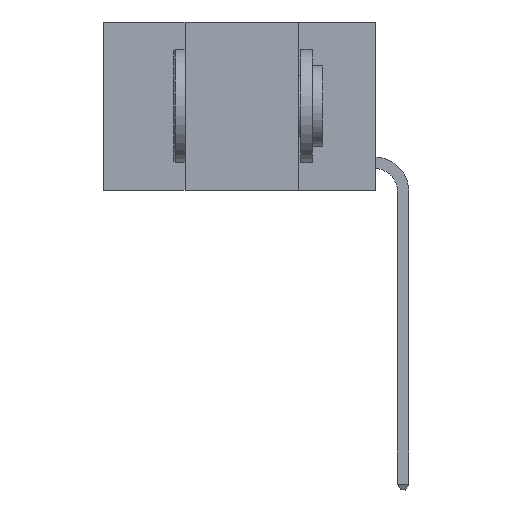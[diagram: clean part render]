
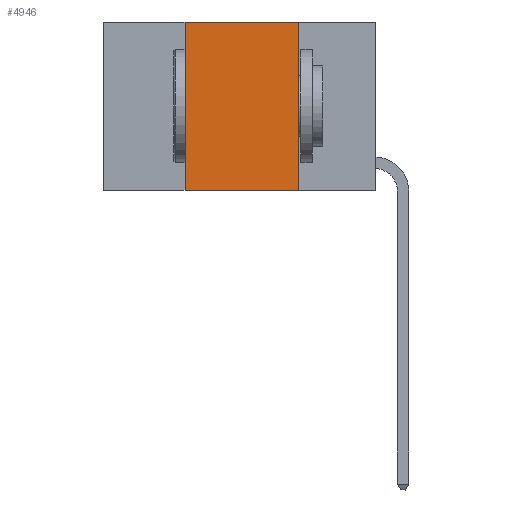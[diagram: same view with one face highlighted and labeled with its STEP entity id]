
A CAD part, left-side view. The second image highlights one B-rep face of the part: STEP entity #4946.
In plain terms, the highlighted planar face has unit normal (-1, 0, 0).
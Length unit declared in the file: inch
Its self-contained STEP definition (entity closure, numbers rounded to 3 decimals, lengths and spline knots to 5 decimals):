
#1655 = CARTESIAN_POINT ( 'NONE',  ( 0., 0.17, 0. ) ) ;
#1860 = AXIS2_PLACEMENT_3D ( 'NONE', #11773, #8439, #4519 ) ;
#2201 = VERTEX_POINT ( 'NONE', #23455 ) ;
#2501 = ORIENTED_EDGE ( 'NONE', *, *, #7021, .F. ) ;
#3033 = DIRECTION ( 'NONE',  ( 0., 0., -1. ) ) ;
#4519 = DIRECTION ( 'NONE',  ( 0., 0., -1. ) ) ;
#4595 = CARTESIAN_POINT ( 'NONE',  ( 0., 0.42, -0.37 ) ) ;
#4626 = FACE_OUTER_BOUND ( 'NONE', #23109, .T. ) ;
#4946 = ADVANCED_FACE ( 'NONE', ( #4626 ), #21467, .F. ) ;
#5181 = VERTEX_POINT ( 'NONE', #4595 ) ;
#6575 = DIRECTION ( 'NONE',  ( 0., -1., 0. ) ) ;
#7021 = EDGE_CURVE ( 'NONE', #2201, #10026, #11549, .T. ) ;
#8439 = DIRECTION ( 'NONE',  ( 1., 0., 0. ) ) ;
#10026 = VERTEX_POINT ( 'NONE', #1655 ) ;
#10428 = LINE ( 'NONE', #23685, #12687 ) ;
#11549 = LINE ( 'NONE', #13533, #18004 ) ;
#11654 = DIRECTION ( 'NONE',  ( 0., -1., 0. ) ) ;
#11773 = CARTESIAN_POINT ( 'NONE',  ( 0., 0.6, 0. ) ) ;
#12687 = VECTOR ( 'NONE', #3033, 39.37008 ) ;
#13533 = CARTESIAN_POINT ( 'NONE',  ( 0., 0.6, 0. ) ) ;
#13561 = VERTEX_POINT ( 'NONE', #16220 ) ;
#15503 = LINE ( 'NONE', #23175, #23399 ) ;
#15741 = VECTOR ( 'NONE', #23298, 39.37008 ) ;
#16220 = CARTESIAN_POINT ( 'NONE',  ( 0., 0.17, -0.37 ) ) ;
#16746 = LINE ( 'NONE', #22428, #15741 ) ;
#16990 = ORIENTED_EDGE ( 'NONE', *, *, #20769, .F. ) ;
#18004 = VECTOR ( 'NONE', #11654, 39.37008 ) ;
#20769 = EDGE_CURVE ( 'NONE', #10026, #13561, #10428, .T. ) ;
#21467 = PLANE ( 'NONE',  #1860 ) ;
#22025 = EDGE_CURVE ( 'NONE', #5181, #13561, #15503, .T. ) ;
#22428 = CARTESIAN_POINT ( 'NONE',  ( 0., 0.42, 0. ) ) ;
#23109 = EDGE_LOOP ( 'NONE', ( #16990, #2501, #23187, #23357 ) ) ;
#23175 = CARTESIAN_POINT ( 'NONE',  ( 0., 0.6, -0.37 ) ) ;
#23187 = ORIENTED_EDGE ( 'NONE', *, *, #23378, .F. ) ;
#23298 = DIRECTION ( 'NONE',  ( 0., 0., 1. ) ) ;
#23357 = ORIENTED_EDGE ( 'NONE', *, *, #22025, .T. ) ;
#23378 = EDGE_CURVE ( 'NONE', #5181, #2201, #16746, .T. ) ;
#23399 = VECTOR ( 'NONE', #6575, 39.37008 ) ;
#23455 = CARTESIAN_POINT ( 'NONE',  ( 0., 0.42, 0. ) ) ;
#23685 = CARTESIAN_POINT ( 'NONE',  ( 0., 0.17, 0. ) ) ;
